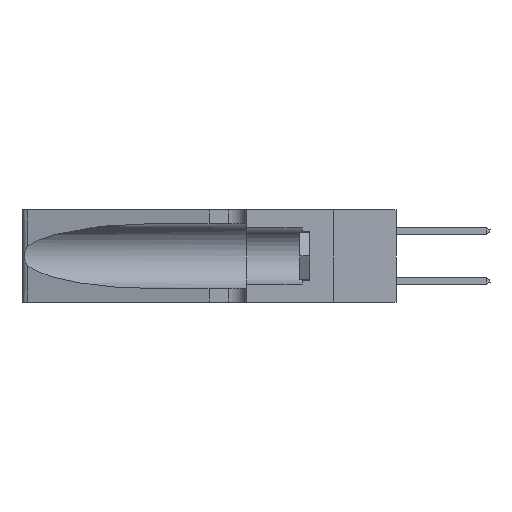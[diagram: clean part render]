
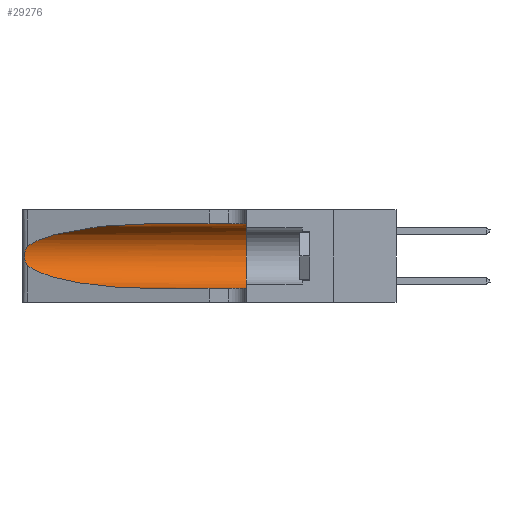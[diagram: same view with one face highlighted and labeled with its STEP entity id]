
A CAD part, left-side view. The second image highlights one B-rep face of the part: STEP entity #29276.
In plain terms, the highlighted cylindrical face has radius 3.308 mm (diameter 6.617 mm), a partial arc.
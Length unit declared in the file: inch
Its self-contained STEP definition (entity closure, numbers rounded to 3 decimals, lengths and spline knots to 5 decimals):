
#242 = CARTESIAN_POINT ( 'NONE',  ( 0.25487, 1.22718, 0.14631 ) ) ;
#391 = CARTESIAN_POINT ( 'NONE',  ( 0.25555, 1.22994, 0.2215 ) ) ;
#1170 = ORIENTED_EDGE ( 'NONE', *, *, #9456, .T. ) ;
#1187 = VERTEX_POINT ( 'NONE', #12871 ) ;
#1445 = DIRECTION ( 'NONE',  ( 0., -1., 0. ) ) ;
#2205 = VERTEX_POINT ( 'NONE', #4556 ) ;
#2340 = CARTESIAN_POINT ( 'NONE',  ( 0.1305, 1.61858, 0.31525 ) ) ;
#3092 = DIRECTION ( 'NONE',  ( 0., -1., 0. ) ) ;
#3480 = AXIS2_PLACEMENT_3D ( 'NONE', #20896, #6504, #42108 ) ;
#3652 = FACE_OUTER_BOUND ( 'NONE', #30606, .T. ) ;
#3788 = CARTESIAN_POINT ( 'NONE',  ( 0.1305, 0.72297, 0.31525 ) ) ;
#3938 = CARTESIAN_POINT ( 'NONE',  ( 0.25639, 1.23186, 0.15144 ) ) ;
#4556 = CARTESIAN_POINT ( 'NONE',  ( 0.1305, 0.35, 0.05475 ) ) ;
#6504 = DIRECTION ( 'NONE',  ( 0., -1., 0. ) ) ;
#7662 = CARTESIAN_POINT ( 'NONE',  ( 0.25487, 1.22718, 0.22369 ) ) ;
#8091 = CYLINDRICAL_SURFACE ( 'NONE', #3480, 0.13025 ) ;
#8951 = ORIENTED_EDGE ( 'NONE', *, *, #12334, .T. ) ;
#9456 = EDGE_CURVE ( 'NONE', #18033, #1187, #43418, .T. ) ;
#9611 = EDGE_CURVE ( 'NONE', #22217, #2205, #23407, .T. ) ;
#12334 = EDGE_CURVE ( 'NONE', #44145, #2205, #15898, .T. ) ;
#12826 = DIRECTION ( 'NONE',  ( 0., 0., 1. ) ) ;
#12871 = CARTESIAN_POINT ( 'NONE',  ( 0.25487, 1.22718, 0.14631 ) ) ;
#14378 = CARTESIAN_POINT ( 'NONE',  ( 0.25487, 1.22718, 0.22369 ) ) ;
#14718 = CARTESIAN_POINT ( 'NONE',  ( 0.25787, 1.23484, 0.2124 ) ) ;
#15898 = LINE ( 'NONE', #22828, #27124 ) ;
#16121 = ORIENTED_EDGE ( 'NONE', *, *, #28789, .T. ) ;
#18033 = VERTEX_POINT ( 'NONE', #21872 ) ;
#18500 = EDGE_CURVE ( 'NONE', #28365, #22217, #28485, .T. ) ;
#20108 = VECTOR ( 'NONE', #3092, 39.37008 ) ;
#20896 = CARTESIAN_POINT ( 'NONE',  ( 0.1305, 1.61858, 0.185 ) ) ;
#21761 = CARTESIAN_POINT ( 'NONE',  ( 0.25854, 1.2359, 0.20912 ) ) ;
#21872 = CARTESIAN_POINT ( 'NONE',  ( 0.25487, 1.22718, 0.22369 ) ) ;
#22055 = CARTESIAN_POINT ( 'NONE',  ( 0.25639, 1.23184, 0.21858 ) ) ;
#22217 = VERTEX_POINT ( 'NONE', #39755 ) ;
#22828 = CARTESIAN_POINT ( 'NONE',  ( 0.1305, 1.61858, 0.05475 ) ) ;
#23407 = CIRCLE ( 'NONE', #25872, 0.13025 ) ;
#23873 = CARTESIAN_POINT ( 'NONE',  ( 0.25487, 1.22718, 0.14631 ) ) ;
#23930 = EDGE_CURVE ( 'NONE', #1187, #44145, #37630, .T. ) ;
#24326 = CARTESIAN_POINT ( 'NONE',  ( 0.2373, 1.15595, 0.08982 ) ) ;
#25194 = CARTESIAN_POINT ( 'NONE',  ( 0.25789, 1.23486, 0.15765 ) ) ;
#25345 = CARTESIAN_POINT ( 'NONE',  ( 0.26075, 1.23896, 0.19203 ) ) ;
#25872 = AXIS2_PLACEMENT_3D ( 'NONE', #34197, #33414, #12826 ) ;
#27124 = VECTOR ( 'NONE', #1445, 39.37008 ) ;
#28365 = VERTEX_POINT ( 'NONE', #3788 ) ;
#28485 = LINE ( 'NONE', #2340, #20108 ) ;
#28588 = CARTESIAN_POINT ( 'NONE',  ( 0.1305, 0.72297, 0.31525 ) ) ;
#28734 = CARTESIAN_POINT ( 'NONE',  ( 0.2373, 1.15595, 0.28018 ) ) ;
#28789 = EDGE_CURVE ( 'NONE', #28365, #18033, #40489, .T. ) ;
#29083 = CARTESIAN_POINT ( 'NONE',  ( 0.26018, 1.23835, 0.19895 ) ) ;
#29276 = ADVANCED_FACE ( 'NONE', ( #3652 ), #8091, .F. ) ;
#30606 = EDGE_LOOP ( 'NONE', ( #16121, #1170, #40332, #8951, #36257, #32359 ) ) ;
#31702 = CARTESIAN_POINT ( 'NONE',  ( 0.18966, 0.96281, 0.31525 ) ) ;
#32359 = ORIENTED_EDGE ( 'NONE', *, *, #18500, .F. ) ;
#33414 = DIRECTION ( 'NONE',  ( 0., 1., 0. ) ) ;
#34197 = CARTESIAN_POINT ( 'NONE',  ( 0.1305, 0.35, 0.185 ) ) ;
#34833 = CARTESIAN_POINT ( 'NONE',  ( 0.1305, 0.72297, 0.05475 ) ) ;
#36257 = ORIENTED_EDGE ( 'NONE', *, *, #9611, .F. ) ;
#37630 =( BOUNDED_CURVE ( )  B_SPLINE_CURVE ( 3, ( #23873, #24326, #42257, #41959 ),
 .UNSPECIFIED., .F., .F. ) 
 B_SPLINE_CURVE_WITH_KNOTS ( ( 4, 4 ),
 ( 3.44316, 4.71239 ),
 .UNSPECIFIED. ) 
 CURVE ( )  GEOMETRIC_REPRESENTATION_ITEM ( )  RATIONAL_B_SPLINE_CURVE ( ( 1., 0.87, 0.87, 1. ) ) 
 REPRESENTATION_ITEM ( '' )  );
#39526 = CARTESIAN_POINT ( 'NONE',  ( 0.26017, 1.23833, 0.17102 ) ) ;
#39755 = CARTESIAN_POINT ( 'NONE',  ( 0.1305, 0.35, 0.31525 ) ) ;
#40332 = ORIENTED_EDGE ( 'NONE', *, *, #23930, .T. ) ;
#40489 =( BOUNDED_CURVE ( )  B_SPLINE_CURVE ( 3, ( #28588, #31702, #28734, #14378 ),
 .UNSPECIFIED., .F., .T. ) 
 B_SPLINE_CURVE_WITH_KNOTS ( ( 4, 4 ),
 ( 1.5708, 2.84003 ),
 .UNSPECIFIED. ) 
 CURVE ( )  GEOMETRIC_REPRESENTATION_ITEM ( )  RATIONAL_B_SPLINE_CURVE ( ( 1., 0.87, 0.87, 1. ) ) 
 REPRESENTATION_ITEM ( '' )  );
#41959 = CARTESIAN_POINT ( 'NONE',  ( 0.1305, 0.72297, 0.05475 ) ) ;
#42108 = DIRECTION ( 'NONE',  ( 0., 0., -1. ) ) ;
#42257 = CARTESIAN_POINT ( 'NONE',  ( 0.18966, 0.96281, 0.05475 ) ) ;
#43133 = CARTESIAN_POINT ( 'NONE',  ( 0.26075, 1.23896, 0.178 ) ) ;
#43289 = CARTESIAN_POINT ( 'NONE',  ( 0.25856, 1.23593, 0.16098 ) ) ;
#43418 = B_SPLINE_CURVE_WITH_KNOTS ( 'NONE', 3,
 ( #7662, #391, #22055, #14718, #21761, #29083, #25345, #43133, #39526, #43289, #25194, #3938, #43448, #242 ),
 .UNSPECIFIED., .F., .F.,
 ( 4, 2, 2, 2, 2, 2, 4 ),
 ( 0., 0.00027, 0.00053, 0.00107, 0.0016, 0.00187, 0.00214 ),
 .UNSPECIFIED. ) ;
#43448 = CARTESIAN_POINT ( 'NONE',  ( 0.25555, 1.22993, 0.14849 ) ) ;
#44145 = VERTEX_POINT ( 'NONE', #34833 ) ;
